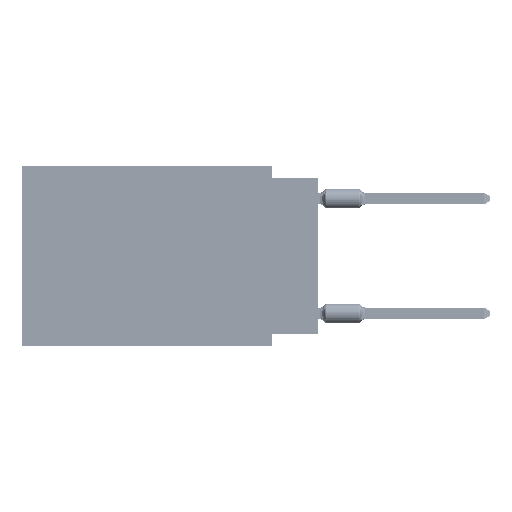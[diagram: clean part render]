
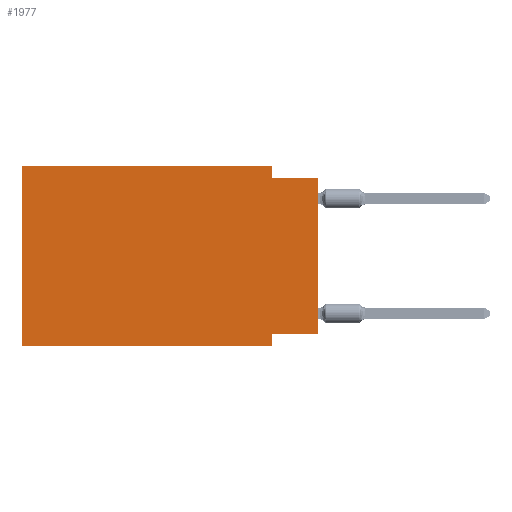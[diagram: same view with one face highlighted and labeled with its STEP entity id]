
A CAD part, left-side view. The second image highlights one B-rep face of the part: STEP entity #1977.
In plain terms, the highlighted planar face has unit normal (-1, 0, 0).
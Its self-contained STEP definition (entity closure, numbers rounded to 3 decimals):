
#626 = DIRECTION ( 'NONE',  ( 0., 0., -1. ) ) ;
#1832 = VECTOR ( 'NONE', #58752, 1000. ) ;
#1977 = ADVANCED_FACE ( 'NONE', ( #32633 ), #46309, .F. ) ;
#4885 = CARTESIAN_POINT ( 'NONE',  ( 0., 0., -9.271 ) ) ;
#5553 = ORIENTED_EDGE ( 'NONE', *, *, #61213, .T. ) ;
#6104 = ORIENTED_EDGE ( 'NONE', *, *, #16844, .F. ) ;
#6185 = CARTESIAN_POINT ( 'NONE',  ( 0., 2.54, 0. ) ) ;
#6407 = EDGE_CURVE ( 'NONE', #30793, #28777, #34429, .T. ) ;
#6774 = LINE ( 'NONE', #27533, #17047 ) ;
#9921 = LINE ( 'NONE', #64644, #43726 ) ;
#12006 = ORIENTED_EDGE ( 'NONE', *, *, #66646, .F. ) ;
#12831 = LINE ( 'NONE', #53439, #1832 ) ;
#12972 = CARTESIAN_POINT ( 'NONE',  ( 0., 0., -9.271 ) ) ;
#14053 = CARTESIAN_POINT ( 'NONE',  ( 0., 16.383, 0. ) ) ;
#14191 = VERTEX_POINT ( 'NONE', #65766 ) ;
#14983 = CARTESIAN_POINT ( 'NONE',  ( 0., 16.383, 0. ) ) ;
#16681 = VERTEX_POINT ( 'NONE', #45513 ) ;
#16844 = EDGE_CURVE ( 'NONE', #28777, #21966, #39271, .T. ) ;
#17047 = VECTOR ( 'NONE', #626, 1000. ) ;
#19055 = CARTESIAN_POINT ( 'NONE',  ( 0., 2.54, -9.906 ) ) ;
#20946 = VECTOR ( 'NONE', #53868, 1000. ) ;
#21966 = VERTEX_POINT ( 'NONE', #45879 ) ;
#22706 = ORIENTED_EDGE ( 'NONE', *, *, #30117, .T. ) ;
#24493 = AXIS2_PLACEMENT_3D ( 'NONE', #14053, #40992, #53362 ) ;
#25233 = ORIENTED_EDGE ( 'NONE', *, *, #76762, .F. ) ;
#25893 = CARTESIAN_POINT ( 'NONE',  ( 0., 16.383, -9.906 ) ) ;
#27533 = CARTESIAN_POINT ( 'NONE',  ( 0., 2.54, -9.906 ) ) ;
#28777 = VERTEX_POINT ( 'NONE', #62784 ) ;
#30117 = EDGE_CURVE ( 'NONE', #33596, #16681, #77425, .T. ) ;
#30793 = VERTEX_POINT ( 'NONE', #69685 ) ;
#31957 = DIRECTION ( 'NONE',  ( 0., 1., 0. ) ) ;
#32633 = FACE_OUTER_BOUND ( 'NONE', #64226, .T. ) ;
#33596 = VERTEX_POINT ( 'NONE', #4885 ) ;
#34429 = LINE ( 'NONE', #14983, #20946 ) ;
#35815 = ORIENTED_EDGE ( 'NONE', *, *, #48377, .F. ) ;
#36846 = DIRECTION ( 'NONE',  ( 0., 0., 1. ) ) ;
#37038 = VECTOR ( 'NONE', #65775, 1000. ) ;
#38299 = ORIENTED_EDGE ( 'NONE', *, *, #57499, .F. ) ;
#39271 = LINE ( 'NONE', #6185, #37038 ) ;
#40992 = DIRECTION ( 'NONE',  ( 1., 0., 0. ) ) ;
#43465 = DIRECTION ( 'NONE',  ( 0., 0., 1. ) ) ;
#43726 = VECTOR ( 'NONE', #36846, 1000. ) ;
#43901 = VERTEX_POINT ( 'NONE', #19055 ) ;
#45513 = CARTESIAN_POINT ( 'NONE',  ( 0., 0., -0.635 ) ) ;
#45879 = CARTESIAN_POINT ( 'NONE',  ( 0., 2.54, -0.635 ) ) ;
#46309 = PLANE ( 'NONE',  #24493 ) ;
#48377 = EDGE_CURVE ( 'NONE', #21966, #16681, #12831, .T. ) ;
#51946 = VECTOR ( 'NONE', #43465, 1000. ) ;
#53362 = DIRECTION ( 'NONE',  ( 0., 0., -1. ) ) ;
#53439 = CARTESIAN_POINT ( 'NONE',  ( 0., 0., -0.635 ) ) ;
#53868 = DIRECTION ( 'NONE',  ( 0., -1., 0. ) ) ;
#55690 = VERTEX_POINT ( 'NONE', #25893 ) ;
#57499 = EDGE_CURVE ( 'NONE', #14191, #43901, #6774, .T. ) ;
#57571 = CARTESIAN_POINT ( 'NONE',  ( 0., 0., 0. ) ) ;
#57815 = ORIENTED_EDGE ( 'NONE', *, *, #6407, .F. ) ;
#58752 = DIRECTION ( 'NONE',  ( 0., -1., 0. ) ) ;
#58796 = LINE ( 'NONE', #78241, #86762 ) ;
#61213 = EDGE_CURVE ( 'NONE', #55690, #43901, #58796, .T. ) ;
#62784 = CARTESIAN_POINT ( 'NONE',  ( 0., 2.54, 0. ) ) ;
#64226 = EDGE_LOOP ( 'NONE', ( #22706, #35815, #6104, #57815, #12006, #5553, #38299, #25233 ) ) ;
#64644 = CARTESIAN_POINT ( 'NONE',  ( 0., 16.383, 0. ) ) ;
#64722 = VECTOR ( 'NONE', #31957, 1000. ) ;
#65524 = LINE ( 'NONE', #12972, #64722 ) ;
#65766 = CARTESIAN_POINT ( 'NONE',  ( 0., 2.54, -9.271 ) ) ;
#65775 = DIRECTION ( 'NONE',  ( 0., 0., -1. ) ) ;
#66646 = EDGE_CURVE ( 'NONE', #55690, #30793, #9921, .T. ) ;
#69685 = CARTESIAN_POINT ( 'NONE',  ( 0., 16.383, 0. ) ) ;
#72051 = DIRECTION ( 'NONE',  ( 0., -1., 0. ) ) ;
#76762 = EDGE_CURVE ( 'NONE', #33596, #14191, #65524, .T. ) ;
#77425 = LINE ( 'NONE', #57571, #51946 ) ;
#78241 = CARTESIAN_POINT ( 'NONE',  ( 0., 16.383, -9.906 ) ) ;
#86762 = VECTOR ( 'NONE', #72051, 1000. ) ;
